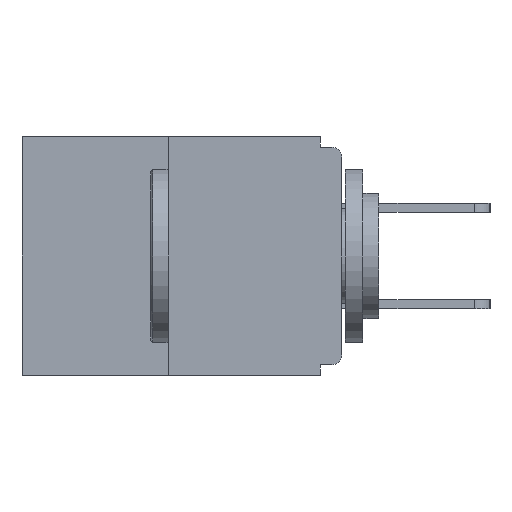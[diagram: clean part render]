
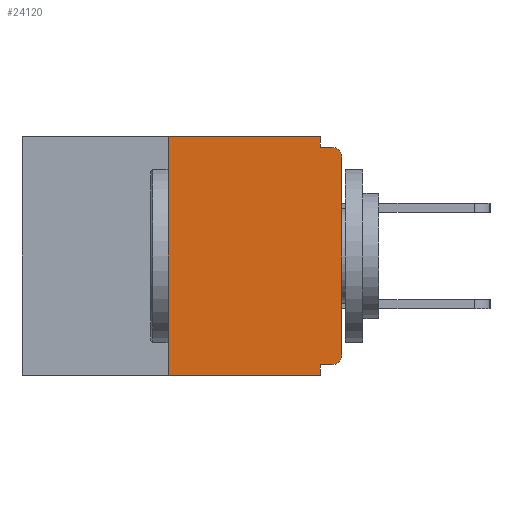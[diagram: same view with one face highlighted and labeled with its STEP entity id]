
A CAD part, left-side view. The second image highlights one B-rep face of the part: STEP entity #24120.
In plain terms, the highlighted planar face has unit normal (-1, 0, 0).
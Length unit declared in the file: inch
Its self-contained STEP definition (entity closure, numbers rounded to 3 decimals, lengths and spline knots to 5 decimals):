
#44 = LINE ( 'NONE', #25720, #15333 ) ;
#1277 = VECTOR ( 'NONE', #27427, 39.37008 ) ;
#1650 = VERTEX_POINT ( 'NONE', #11842 ) ;
#1662 = VERTEX_POINT ( 'NONE', #18037 ) ;
#1734 = FACE_OUTER_BOUND ( 'NONE', #16643, .T. ) ;
#3506 = CARTESIAN_POINT ( 'NONE',  ( 0., 0.015, -0.328 ) ) ;
#3797 = DIRECTION ( 'NONE',  ( 0., 0., -1. ) ) ;
#3869 = CARTESIAN_POINT ( 'NONE',  ( 0., 0.46, 0. ) ) ;
#3958 = DIRECTION ( 'NONE',  ( 0., -1., 0. ) ) ;
#4294 = LINE ( 'NONE', #5420, #29377 ) ;
#4341 = VERTEX_POINT ( 'NONE', #19707 ) ;
#4954 = DIRECTION ( 'NONE',  ( 0., 0., 1. ) ) ;
#5045 = AXIS2_PLACEMENT_3D ( 'NONE', #14568, #14369, #5112 ) ;
#5112 = DIRECTION ( 'NONE',  ( 0., 0., -1. ) ) ;
#5345 = AXIS2_PLACEMENT_3D ( 'NONE', #24669, #17613, #3797 ) ;
#5420 = CARTESIAN_POINT ( 'NONE',  ( 0., 0.031, 0. ) ) ;
#5535 = EDGE_CURVE ( 'NONE', #15000, #4341, #22901, .T. ) ;
#5709 = DIRECTION ( 'NONE',  ( 0., 0., -1. ) ) ;
#5894 = DIRECTION ( 'NONE',  ( 0., 0., -1. ) ) ;
#6327 = VERTEX_POINT ( 'NONE', #12671 ) ;
#6562 = PLANE ( 'NONE',  #12804 ) ;
#7247 = VECTOR ( 'NONE', #10177, 39.37008 ) ;
#8809 = CARTESIAN_POINT ( 'NONE',  ( 0., 0.46, 0. ) ) ;
#9318 = VECTOR ( 'NONE', #12363, 39.37008 ) ;
#9565 = EDGE_CURVE ( 'NONE', #4341, #9776, #25556, .T. ) ;
#9766 = ORIENTED_EDGE ( 'NONE', *, *, #27224, .F. ) ;
#9776 = VERTEX_POINT ( 'NONE', #29794 ) ;
#10177 = DIRECTION ( 'NONE',  ( 0., -1., 0. ) ) ;
#10209 = VERTEX_POINT ( 'NONE', #20354 ) ;
#10439 = CARTESIAN_POINT ( 'NONE',  ( 0., 0.031, -0.328 ) ) ;
#10644 = ORIENTED_EDGE ( 'NONE', *, *, #20129, .F. ) ;
#10661 = CARTESIAN_POINT ( 'NONE',  ( 0., 0., -0.328 ) ) ;
#11359 = ORIENTED_EDGE ( 'NONE', *, *, #29463, .T. ) ;
#11389 = ORIENTED_EDGE ( 'NONE', *, *, #15770, .T. ) ;
#11842 = CARTESIAN_POINT ( 'NONE',  ( 0., 0.25, -0.343 ) ) ;
#12363 = DIRECTION ( 'NONE',  ( 0., -1., 0. ) ) ;
#12418 = CARTESIAN_POINT ( 'NONE',  ( 0., 0.031, -0.343 ) ) ;
#12671 = CARTESIAN_POINT ( 'NONE',  ( 0., 0.031, -0.015 ) ) ;
#12804 = AXIS2_PLACEMENT_3D ( 'NONE', #8809, #22609, #27336 ) ;
#13711 = CARTESIAN_POINT ( 'NONE',  ( 0., 0.25, 0. ) ) ;
#13960 = ORIENTED_EDGE ( 'NONE', *, *, #5535, .T. ) ;
#14369 = DIRECTION ( 'NONE',  ( -1., 0., 0. ) ) ;
#14495 = CIRCLE ( 'NONE', #5345, 0.015 ) ;
#14568 = CARTESIAN_POINT ( 'NONE',  ( 0., 0.015, -0.03 ) ) ;
#14590 = LINE ( 'NONE', #12418, #20448 ) ;
#14668 = ORIENTED_EDGE ( 'NONE', *, *, #18177, .F. ) ;
#15000 = VERTEX_POINT ( 'NONE', #20130 ) ;
#15333 = VECTOR ( 'NONE', #4954, 39.37008 ) ;
#15770 = EDGE_CURVE ( 'NONE', #1650, #1662, #17106, .T. ) ;
#16643 = EDGE_LOOP ( 'NONE', ( #16809, #9766, #11389, #10644, #14668, #11359, #13960, #18983, #23471, #28115 ) ) ;
#16809 = ORIENTED_EDGE ( 'NONE', *, *, #26976, .F. ) ;
#17106 = LINE ( 'NONE', #29134, #7247 ) ;
#17523 = VECTOR ( 'NONE', #3958, 39.37008 ) ;
#17613 = DIRECTION ( 'NONE',  ( -1., 0., 0. ) ) ;
#17997 = EDGE_CURVE ( 'NONE', #10209, #6327, #4294, .T. ) ;
#18037 = CARTESIAN_POINT ( 'NONE',  ( 0., 0.031, -0.343 ) ) ;
#18177 = EDGE_CURVE ( 'NONE', #22352, #23948, #25966, .T. ) ;
#18471 = CARTESIAN_POINT ( 'NONE',  ( 0., 0., 0. ) ) ;
#18686 = DIRECTION ( 'NONE',  ( 0., 1., 0. ) ) ;
#18983 = ORIENTED_EDGE ( 'NONE', *, *, #9565, .T. ) ;
#19707 = CARTESIAN_POINT ( 'NONE',  ( 0., 0., -0.03 ) ) ;
#20129 = EDGE_CURVE ( 'NONE', #23948, #1662, #14590, .T. ) ;
#20130 = CARTESIAN_POINT ( 'NONE',  ( 0., 0., -0.313 ) ) ;
#20354 = CARTESIAN_POINT ( 'NONE',  ( 0., 0.031, 0. ) ) ;
#20448 = VECTOR ( 'NONE', #5894, 39.37008 ) ;
#22352 = VERTEX_POINT ( 'NONE', #3506 ) ;
#22609 = DIRECTION ( 'NONE',  ( 1., 0., 0. ) ) ;
#22723 = EDGE_CURVE ( 'NONE', #6327, #9776, #22849, .T. ) ;
#22849 = LINE ( 'NONE', #28839, #9318 ) ;
#22901 = LINE ( 'NONE', #18471, #1277 ) ;
#23471 = ORIENTED_EDGE ( 'NONE', *, *, #22723, .F. ) ;
#23766 = LINE ( 'NONE', #3869, #17523 ) ;
#23948 = VERTEX_POINT ( 'NONE', #10439 ) ;
#24120 = ADVANCED_FACE ( 'NONE', ( #1734 ), #6562, .F. ) ;
#24531 = VECTOR ( 'NONE', #18686, 39.37008 ) ;
#24669 = CARTESIAN_POINT ( 'NONE',  ( 0., 0.015, -0.313 ) ) ;
#25556 = CIRCLE ( 'NONE', #5045, 0.015 ) ;
#25720 = CARTESIAN_POINT ( 'NONE',  ( 0., 0.25, 0. ) ) ;
#25966 = LINE ( 'NONE', #10661, #24531 ) ;
#26976 = EDGE_CURVE ( 'NONE', #27022, #10209, #23766, .T. ) ;
#27022 = VERTEX_POINT ( 'NONE', #13711 ) ;
#27224 = EDGE_CURVE ( 'NONE', #1650, #27022, #44, .T. ) ;
#27336 = DIRECTION ( 'NONE',  ( 0., 0., -1. ) ) ;
#27427 = DIRECTION ( 'NONE',  ( 0., 0., 1. ) ) ;
#28115 = ORIENTED_EDGE ( 'NONE', *, *, #17997, .F. ) ;
#28839 = CARTESIAN_POINT ( 'NONE',  ( 0., 0., -0.015 ) ) ;
#29134 = CARTESIAN_POINT ( 'NONE',  ( 0., 0.46, -0.343 ) ) ;
#29377 = VECTOR ( 'NONE', #5709, 39.37008 ) ;
#29463 = EDGE_CURVE ( 'NONE', #22352, #15000, #14495, .T. ) ;
#29794 = CARTESIAN_POINT ( 'NONE',  ( 0., 0.015, -0.015 ) ) ;
